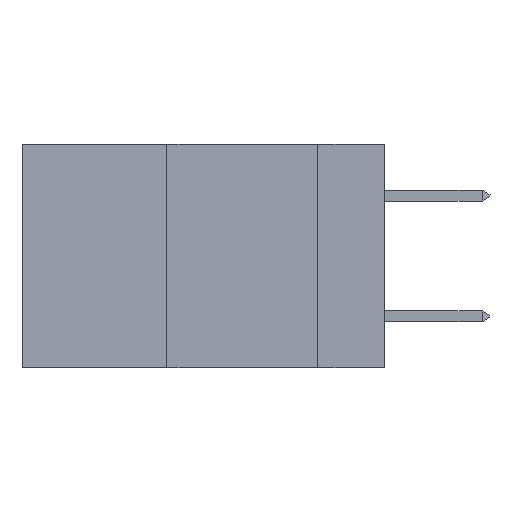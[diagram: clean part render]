
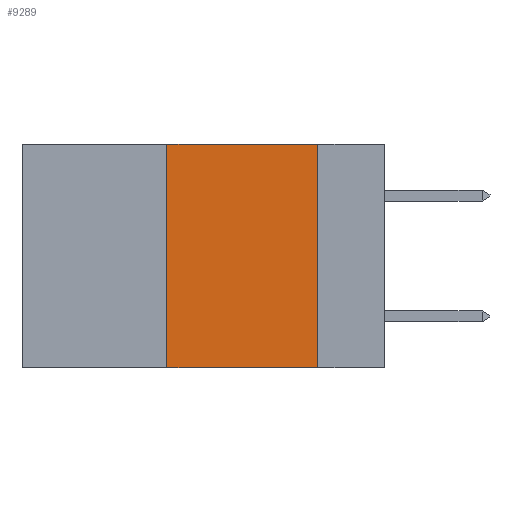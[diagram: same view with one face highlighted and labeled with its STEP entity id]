
A CAD part, left-side view. The second image highlights one B-rep face of the part: STEP entity #9289.
In plain terms, the highlighted planar face has unit normal (-1, 0, 0).
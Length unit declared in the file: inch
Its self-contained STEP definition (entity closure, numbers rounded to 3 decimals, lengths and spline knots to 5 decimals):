
#10 = PLANE ( 'NONE',  #2870 ) ;
#249 = DIRECTION ( 'NONE',  ( 0., 0., -1. ) ) ;
#302 = CARTESIAN_POINT ( 'NONE',  ( 0., 0.6, 0. ) ) ;
#624 = VECTOR ( 'NONE', #12532, 39.37008 ) ;
#803 = EDGE_CURVE ( 'NONE', #4339, #1603, #2687, .T. ) ;
#1300 = CARTESIAN_POINT ( 'NONE',  ( 0., 0.36, 0. ) ) ;
#1603 = VERTEX_POINT ( 'NONE', #1643 ) ;
#1643 = CARTESIAN_POINT ( 'NONE',  ( 0., 0.36, 0. ) ) ;
#1930 = VECTOR ( 'NONE', #249, 39.37008 ) ;
#2260 = CARTESIAN_POINT ( 'NONE',  ( 0., 0.36, -0.37 ) ) ;
#2687 = LINE ( 'NONE', #1300, #624 ) ;
#2698 = EDGE_CURVE ( 'NONE', #1603, #10828, #10774, .T. ) ;
#2870 = AXIS2_PLACEMENT_3D ( 'NONE', #9260, #3097, #10238 ) ;
#3097 = DIRECTION ( 'NONE',  ( 1., 0., 0. ) ) ;
#4339 = VERTEX_POINT ( 'NONE', #2260 ) ;
#4428 = ORIENTED_EDGE ( 'NONE', *, *, #11599, .F. ) ;
#4525 = DIRECTION ( 'NONE',  ( 0., -1., 0. ) ) ;
#4778 = EDGE_LOOP ( 'NONE', ( #4428, #7465, #11969, #12082 ) ) ;
#5454 = VECTOR ( 'NONE', #4525, 39.37008 ) ;
#5615 = DIRECTION ( 'NONE',  ( 0., -1., 0. ) ) ;
#6993 = EDGE_CURVE ( 'NONE', #4339, #8881, #9639, .T. ) ;
#7460 = LINE ( 'NONE', #12340, #1930 ) ;
#7465 = ORIENTED_EDGE ( 'NONE', *, *, #2698, .F. ) ;
#7701 = FACE_OUTER_BOUND ( 'NONE', #4778, .T. ) ;
#8278 = CARTESIAN_POINT ( 'NONE',  ( 0., 0.11, 0. ) ) ;
#8881 = VERTEX_POINT ( 'NONE', #11512 ) ;
#9260 = CARTESIAN_POINT ( 'NONE',  ( 0., 0.6, 0. ) ) ;
#9289 = ADVANCED_FACE ( 'NONE', ( #7701 ), #10, .F. ) ;
#9321 = VECTOR ( 'NONE', #5615, 39.37008 ) ;
#9639 = LINE ( 'NONE', #12527, #9321 ) ;
#10238 = DIRECTION ( 'NONE',  ( 0., 0., -1. ) ) ;
#10774 = LINE ( 'NONE', #302, #5454 ) ;
#10828 = VERTEX_POINT ( 'NONE', #8278 ) ;
#11512 = CARTESIAN_POINT ( 'NONE',  ( 0., 0.11, -0.37 ) ) ;
#11599 = EDGE_CURVE ( 'NONE', #10828, #8881, #7460, .T. ) ;
#11969 = ORIENTED_EDGE ( 'NONE', *, *, #803, .F. ) ;
#12082 = ORIENTED_EDGE ( 'NONE', *, *, #6993, .T. ) ;
#12340 = CARTESIAN_POINT ( 'NONE',  ( 0., 0.11, 0. ) ) ;
#12527 = CARTESIAN_POINT ( 'NONE',  ( 0., 0.6, -0.37 ) ) ;
#12532 = DIRECTION ( 'NONE',  ( 0., 0., 1. ) ) ;
